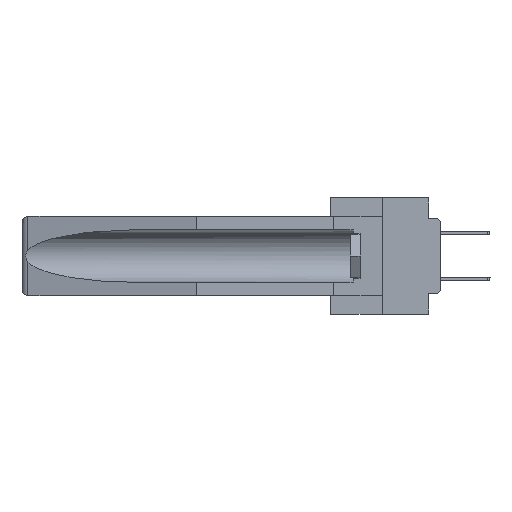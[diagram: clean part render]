
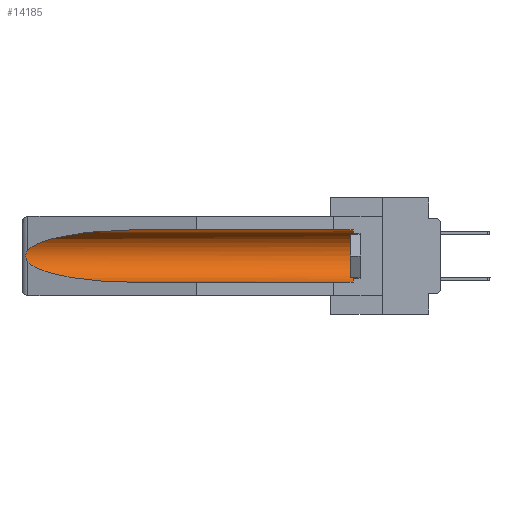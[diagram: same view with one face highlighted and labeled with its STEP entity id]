
A CAD part, left-side view. The second image highlights one B-rep face of the part: STEP entity #14185.
In plain terms, the highlighted cylindrical face has radius 2.857 mm (diameter 5.715 mm), a partial arc.
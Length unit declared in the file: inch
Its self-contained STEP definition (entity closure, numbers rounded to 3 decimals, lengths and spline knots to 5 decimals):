
#321 = CARTESIAN_POINT ( 'NONE',  ( 0.25451, 1.48313, -0.24835 ) ) ;
#924 = ORIENTED_EDGE ( 'NONE', *, *, #8012, .T. ) ;
#1357 = CARTESIAN_POINT ( 'NONE',  ( 0.26537, 1.52718, -0.14972 ) ) ;
#1492 = CARTESIAN_POINT ( 'NONE',  ( 0.2673, 1.5327, -0.16383 ) ) ;
#1803 = CARTESIAN_POINT ( 'NONE',  ( 0.26537, 1.52718, -0.19328 ) ) ;
#2013 = CIRCLE ( 'NONE', #34960, 0.1125 ) ;
#2303 = CARTESIAN_POINT ( 'NONE',  ( 0.26537, 1.52718, -0.14972 ) ) ;
#2632 = CARTESIAN_POINT ( 'NONE',  ( 0.155, 1.07973, -0.284 ) ) ;
#3625 = CARTESIAN_POINT ( 'NONE',  ( 0.26537, 1.52718, -0.19328 ) ) ;
#4060 = CARTESIAN_POINT ( 'NONE',  ( 0.25451, 1.48313, -0.09465 ) ) ;
#4420 = CARTESIAN_POINT ( 'NONE',  ( 0.2673, 1.53269, -0.17917 ) ) ;
#4444 = CARTESIAN_POINT ( 'NONE',  ( 0.155, 1.07973, -0.059 ) ) ;
#5163 = DIRECTION ( 'NONE',  ( 0., 1., 0. ) ) ;
#5294 = LINE ( 'NONE', #30993, #12983 ) ;
#5652 = CARTESIAN_POINT ( 'NONE',  ( 0.155, 1.07973, -0.059 ) ) ;
#5976 =( BOUNDED_CURVE ( )  B_SPLINE_CURVE ( 3, ( #3625, #321, #20544, #29547 ),
 .UNSPECIFIED., .F., .F. ) 
 B_SPLINE_CURVE_WITH_KNOTS ( ( 4, 4 ),
 ( 0.1948, 1.5708 ),
 .UNSPECIFIED. ) 
 CURVE ( )  GEOMETRIC_REPRESENTATION_ITEM ( )  RATIONAL_B_SPLINE_CURVE ( ( 1., 0.848, 0.848, 1. ) ) 
 REPRESENTATION_ITEM ( '' )  );
#7651 = VERTEX_POINT ( 'NONE', #33606 ) ;
#8012 = EDGE_CURVE ( 'NONE', #18292, #28191, #8752, .T. ) ;
#8752 =( BOUNDED_CURVE ( )  B_SPLINE_CURVE ( 3, ( #4444, #29395, #4060, #2303 ),
 .UNSPECIFIED., .F., .F. ) 
 B_SPLINE_CURVE_WITH_KNOTS ( ( 4, 4 ),
 ( 4.71239, 6.08839 ),
 .UNSPECIFIED. ) 
 CURVE ( )  GEOMETRIC_REPRESENTATION_ITEM ( )  RATIONAL_B_SPLINE_CURVE ( ( 1., 0.848, 0.848, 1. ) ) 
 REPRESENTATION_ITEM ( '' )  );
#9063 = ORIENTED_EDGE ( 'NONE', *, *, #11061, .T. ) ;
#9492 = DIRECTION ( 'NONE',  ( 0., -1., 0. ) ) ;
#9506 = ORIENTED_EDGE ( 'NONE', *, *, #11989, .F. ) ;
#9627 = CYLINDRICAL_SURFACE ( 'NONE', #25230, 0.1125 ) ;
#10868 = CARTESIAN_POINT ( 'NONE',  ( 0.155, -0.30754, -0.059 ) ) ;
#11061 = EDGE_CURVE ( 'NONE', #34803, #18292, #15728, .T. ) ;
#11989 = EDGE_CURVE ( 'NONE', #7651, #29699, #5294, .T. ) ;
#12983 = VECTOR ( 'NONE', #5163, 39.37008 ) ;
#13526 = DIRECTION ( 'NONE',  ( 0., 1., 0. ) ) ;
#13900 = EDGE_CURVE ( 'NONE', #7651, #34803, #2013, .T. ) ;
#14185 = ADVANCED_FACE ( 'NONE', ( #26749 ), #9627, .F. ) ;
#14832 = CARTESIAN_POINT ( 'NONE',  ( 0.155, 0.126, -0.1715 ) ) ;
#15660 = CARTESIAN_POINT ( 'NONE',  ( 0.26597, 1.5296, -0.19026 ) ) ;
#15728 = LINE ( 'NONE', #10868, #21589 ) ;
#16989 = CARTESIAN_POINT ( 'NONE',  ( 0.155, -0.30754, -0.1715 ) ) ;
#17494 = EDGE_CURVE ( 'NONE', #28191, #23104, #24291, .T. ) ;
#17955 = DIRECTION ( 'NONE',  ( 0., 0., 1. ) ) ;
#18292 = VERTEX_POINT ( 'NONE', #5652 ) ;
#18333 = ORIENTED_EDGE ( 'NONE', *, *, #13900, .T. ) ;
#18407 = CARTESIAN_POINT ( 'NONE',  ( 0.26655, 1.53094, -0.18657 ) ) ;
#20536 = CARTESIAN_POINT ( 'NONE',  ( 0.26537, 1.52718, -0.14972 ) ) ;
#20544 = CARTESIAN_POINT ( 'NONE',  ( 0.21114, 1.30732, -0.284 ) ) ;
#20929 = ORIENTED_EDGE ( 'NONE', *, *, #17494, .T. ) ;
#21589 = VECTOR ( 'NONE', #13526, 39.37008 ) ;
#21730 = CARTESIAN_POINT ( 'NONE',  ( 0.2675, 1.53308, -0.17534 ) ) ;
#22397 = ORIENTED_EDGE ( 'NONE', *, *, #24495, .T. ) ;
#23104 = VERTEX_POINT ( 'NONE', #1803 ) ;
#23153 = DIRECTION ( 'NONE',  ( 0., 1., 0. ) ) ;
#24291 = B_SPLINE_CURVE_WITH_KNOTS ( 'NONE', 3,
 ( #1357, #27243, #32894, #1492, #30210, #21730, #4420, #18407, #15660, #24644 ),
 .UNSPECIFIED., .F., .F.,
 ( 4, 2, 2, 2, 4 ),
 ( 0., 0.00029, 0.00058, 0.00087, 0.00117 ),
 .UNSPECIFIED. ) ;
#24495 = EDGE_CURVE ( 'NONE', #23104, #29699, #5976, .T. ) ;
#24644 = CARTESIAN_POINT ( 'NONE',  ( 0.26537, 1.52718, -0.19328 ) ) ;
#25230 = AXIS2_PLACEMENT_3D ( 'NONE', #16989, #23153, #29209 ) ;
#26749 = FACE_OUTER_BOUND ( 'NONE', #35705, .T. ) ;
#27243 = CARTESIAN_POINT ( 'NONE',  ( 0.26597, 1.52961, -0.15275 ) ) ;
#28191 = VERTEX_POINT ( 'NONE', #20536 ) ;
#29209 = DIRECTION ( 'NONE',  ( 0., 0., 1. ) ) ;
#29395 = CARTESIAN_POINT ( 'NONE',  ( 0.21114, 1.30732, -0.059 ) ) ;
#29547 = CARTESIAN_POINT ( 'NONE',  ( 0.155, 1.07973, -0.284 ) ) ;
#29699 = VERTEX_POINT ( 'NONE', #2632 ) ;
#30181 = CARTESIAN_POINT ( 'NONE',  ( 0.155, 0.126, -0.059 ) ) ;
#30210 = CARTESIAN_POINT ( 'NONE',  ( 0.2675, 1.53308, -0.16763 ) ) ;
#30993 = CARTESIAN_POINT ( 'NONE',  ( 0.155, -0.30754, -0.284 ) ) ;
#32894 = CARTESIAN_POINT ( 'NONE',  ( 0.26654, 1.53092, -0.15636 ) ) ;
#33606 = CARTESIAN_POINT ( 'NONE',  ( 0.155, 0.126, -0.284 ) ) ;
#34803 = VERTEX_POINT ( 'NONE', #30181 ) ;
#34960 = AXIS2_PLACEMENT_3D ( 'NONE', #14832, #9492, #17955 ) ;
#35705 = EDGE_LOOP ( 'NONE', ( #924, #20929, #22397, #9506, #18333, #9063 ) ) ;
